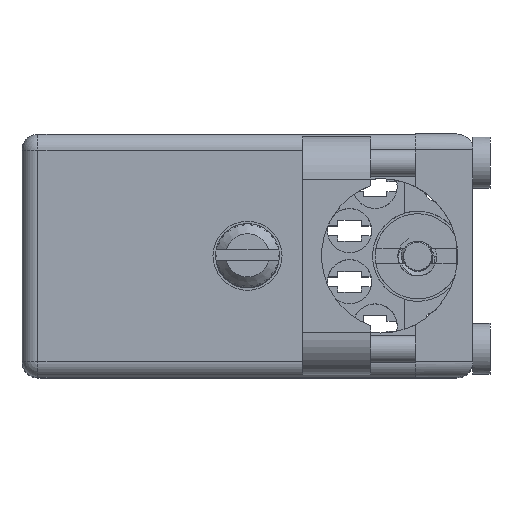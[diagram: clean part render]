
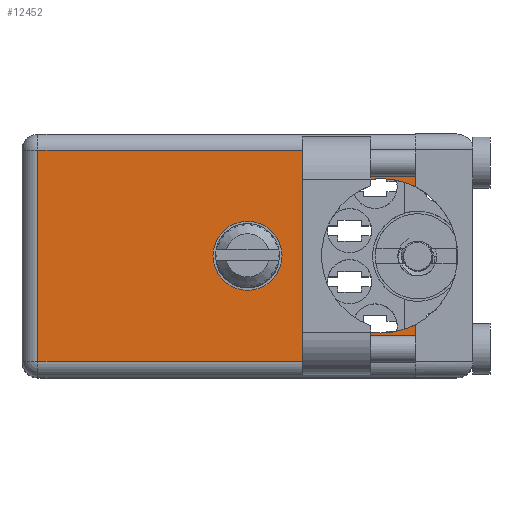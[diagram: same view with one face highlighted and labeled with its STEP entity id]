
A CAD part, top view. The second image highlights one B-rep face of the part: STEP entity #12452.
In plain terms, the highlighted face is planar.
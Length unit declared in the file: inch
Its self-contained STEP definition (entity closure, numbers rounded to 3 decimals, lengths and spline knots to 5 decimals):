
#3564 = AXIS2_PLACEMENT_3D ( 'NONE', #64339, #185907, #63037 ) ;
#4004 = ORIENTED_EDGE ( 'NONE', *, *, #131707, .F. ) ;
#4763 = CIRCLE ( 'NONE', #82189, 0.227 ) ;
#12452 = ADVANCED_FACE ( 'NONE', ( #127771, #182117 ), #57680, .T. ) ;
#15146 = CARTESIAN_POINT ( 'NONE',  ( 0., 0.806, 0.1015 ) ) ;
#22036 = CARTESIAN_POINT ( 'NONE',  ( 0.4925, 0.806, 0.3105 ) ) ;
#23377 = VERTEX_POINT ( 'NONE', #166160 ) ;
#24652 = VERTEX_POINT ( 'NONE', #145278 ) ;
#24810 = CARTESIAN_POINT ( 'NONE',  ( 0., 0.806, -0.1015 ) ) ;
#26362 = VERTEX_POINT ( 'NONE', #117963 ) ;
#27257 = DIRECTION ( 'NONE',  ( 0., 0., 1. ) ) ;
#27502 = EDGE_CURVE ( 'NONE', #118082, #26362, #44327, .T. ) ;
#32423 = ORIENTED_EDGE ( 'NONE', *, *, #138643, .F. ) ;
#33767 = VERTEX_POINT ( 'NONE', #22036 ) ;
#34759 = EDGE_CURVE ( 'NONE', #118082, #40031, #74350, .T. ) ;
#36095 = DIRECTION ( 'NONE',  ( 1., 0., 0. ) ) ;
#36888 = CARTESIAN_POINT ( 'NONE',  ( -0.6155, 0.806, 0.3105 ) ) ;
#39247 = EDGE_LOOP ( 'NONE', ( #73525, #182724 ) ) ;
#40031 = VERTEX_POINT ( 'NONE', #142792 ) ;
#42899 = EDGE_CURVE ( 'NONE', #26362, #23377, #75351, .T. ) ;
#43878 = LINE ( 'NONE', #112731, #102999 ) ;
#44327 = LINE ( 'NONE', #161524, #157962 ) ;
#45729 = CARTESIAN_POINT ( 'NONE',  ( 0.4925, 0.806, 0.20279 ) ) ;
#48483 = DIRECTION ( 'NONE',  ( 0., 0., 1. ) ) ;
#52326 = VECTOR ( 'NONE', #27257, 39.37008 ) ;
#56157 = DIRECTION ( 'NONE',  ( 0., 1., 0. ) ) ;
#57680 = PLANE ( 'NONE',  #170987 ) ;
#58452 = ORIENTED_EDGE ( 'NONE', *, *, #27502, .F. ) ;
#62411 = CARTESIAN_POINT ( 'NONE',  ( 0.4925, 0.806, -0.3105 ) ) ;
#63037 = DIRECTION ( 'NONE',  ( -1., 0., 0. ) ) ;
#64339 = CARTESIAN_POINT ( 'NONE',  ( 0.3905, 0.806, 0. ) ) ;
#67726 = ORIENTED_EDGE ( 'NONE', *, *, #34759, .T. ) ;
#70134 = VERTEX_POINT ( 'NONE', #15146 ) ;
#72011 = DIRECTION ( 'NONE',  ( -1., 0., 0. ) ) ;
#73525 = ORIENTED_EDGE ( 'NONE', *, *, #193565, .F. ) ;
#74350 = LINE ( 'NONE', #107620, #157074 ) ;
#75351 = CIRCLE ( 'NONE', #102804, 0.227 ) ;
#75997 = VERTEX_POINT ( 'NONE', #24810 ) ;
#76588 = DIRECTION ( 'NONE',  ( -1., 0., 0. ) ) ;
#77615 = DIRECTION ( 'NONE',  ( 0., 1., 0. ) ) ;
#79307 = LINE ( 'NONE', #181074, #187953 ) ;
#80412 = CARTESIAN_POINT ( 'NONE',  ( 0.3905, 0.806, 0. ) ) ;
#82189 = AXIS2_PLACEMENT_3D ( 'NONE', #80412, #157067, #186102 ) ;
#82645 = VERTEX_POINT ( 'NONE', #36888 ) ;
#85056 = EDGE_CURVE ( 'NONE', #82645, #33767, #43878, .T. ) ;
#90093 = DIRECTION ( 'NONE',  ( -1., 0., 0. ) ) ;
#95807 = CIRCLE ( 'NONE', #3564, 0.227 ) ;
#97111 = DIRECTION ( 'NONE',  ( 0., 0., 1. ) ) ;
#98913 = EDGE_LOOP ( 'NONE', ( #58452, #67726, #174896, #139787, #137061, #4004, #32423, #127423 ) ) ;
#99078 = AXIS2_PLACEMENT_3D ( 'NONE', #110644, #77615, #48483 ) ;
#102804 = AXIS2_PLACEMENT_3D ( 'NONE', #118917, #56157, #72011 ) ;
#102999 = VECTOR ( 'NONE', #36095, 39.37008 ) ;
#103163 = CIRCLE ( 'NONE', #99078, 0.1015 ) ;
#107620 = CARTESIAN_POINT ( 'NONE',  ( -0.6625, 0.806, -0.3105 ) ) ;
#110644 = CARTESIAN_POINT ( 'NONE',  ( 0., 0.806, 0. ) ) ;
#112731 = CARTESIAN_POINT ( 'NONE',  ( 0.4925, 0.806, 0.3105 ) ) ;
#114156 = AXIS2_PLACEMENT_3D ( 'NONE', #159851, #174441, #97111 ) ;
#117963 = CARTESIAN_POINT ( 'NONE',  ( 0.4925, 0.806, -0.20279 ) ) ;
#118082 = VERTEX_POINT ( 'NONE', #62411 ) ;
#118917 = CARTESIAN_POINT ( 'NONE',  ( 0.3905, 0.806, 0. ) ) ;
#119516 = VERTEX_POINT ( 'NONE', #45729 ) ;
#127423 = ORIENTED_EDGE ( 'NONE', *, *, #42899, .F. ) ;
#127771 = FACE_OUTER_BOUND ( 'NONE', #98913, .T. ) ;
#131707 = EDGE_CURVE ( 'NONE', #24652, #119516, #95807, .T. ) ;
#132310 = CARTESIAN_POINT ( 'NONE',  ( -0.6155, 0.806, -0.3575 ) ) ;
#135656 = CARTESIAN_POINT ( 'NONE',  ( -0.6625, 0.806, -0.3575 ) ) ;
#137061 = ORIENTED_EDGE ( 'NONE', *, *, #174457, .F. ) ;
#138643 = EDGE_CURVE ( 'NONE', #23377, #24652, #4763, .T. ) ;
#139787 = ORIENTED_EDGE ( 'NONE', *, *, #85056, .T. ) ;
#142792 = CARTESIAN_POINT ( 'NONE',  ( -0.6155, 0.806, -0.3105 ) ) ;
#145278 = CARTESIAN_POINT ( 'NONE',  ( 0.3905, 0.806, 0.227 ) ) ;
#146295 = DIRECTION ( 'NONE',  ( 0., 0., 1. ) ) ;
#157067 = DIRECTION ( 'NONE',  ( 0., 1., 0. ) ) ;
#157074 = VECTOR ( 'NONE', #76588, 39.37008 ) ;
#157962 = VECTOR ( 'NONE', #146295, 39.37008 ) ;
#159851 = CARTESIAN_POINT ( 'NONE',  ( 0., 0.806, 0. ) ) ;
#161165 = LINE ( 'NONE', #132310, #52326 ) ;
#161524 = CARTESIAN_POINT ( 'NONE',  ( 0.4925, 0.806, 0.3575 ) ) ;
#164066 = DIRECTION ( 'NONE',  ( 0., 1., 0. ) ) ;
#164545 = CIRCLE ( 'NONE', #114156, 0.1015 ) ;
#166160 = CARTESIAN_POINT ( 'NONE',  ( 0.3905, 0.806, -0.227 ) ) ;
#166493 = DIRECTION ( 'NONE',  ( 0., 0., 1. ) ) ;
#170987 = AXIS2_PLACEMENT_3D ( 'NONE', #135656, #164066, #90093 ) ;
#174441 = DIRECTION ( 'NONE',  ( 0., 1., 0. ) ) ;
#174457 = EDGE_CURVE ( 'NONE', #119516, #33767, #79307, .T. ) ;
#174896 = ORIENTED_EDGE ( 'NONE', *, *, #186117, .T. ) ;
#181074 = CARTESIAN_POINT ( 'NONE',  ( 0.4925, 0.806, 0.3575 ) ) ;
#182117 = FACE_BOUND ( 'NONE', #39247, .T. ) ;
#182724 = ORIENTED_EDGE ( 'NONE', *, *, #194185, .F. ) ;
#185907 = DIRECTION ( 'NONE',  ( 0., 1., 0. ) ) ;
#186102 = DIRECTION ( 'NONE',  ( -1., 0., 0. ) ) ;
#186117 = EDGE_CURVE ( 'NONE', #40031, #82645, #161165, .T. ) ;
#187953 = VECTOR ( 'NONE', #166493, 39.37008 ) ;
#193565 = EDGE_CURVE ( 'NONE', #70134, #75997, #164545, .T. ) ;
#194185 = EDGE_CURVE ( 'NONE', #75997, #70134, #103163, .T. ) ;
